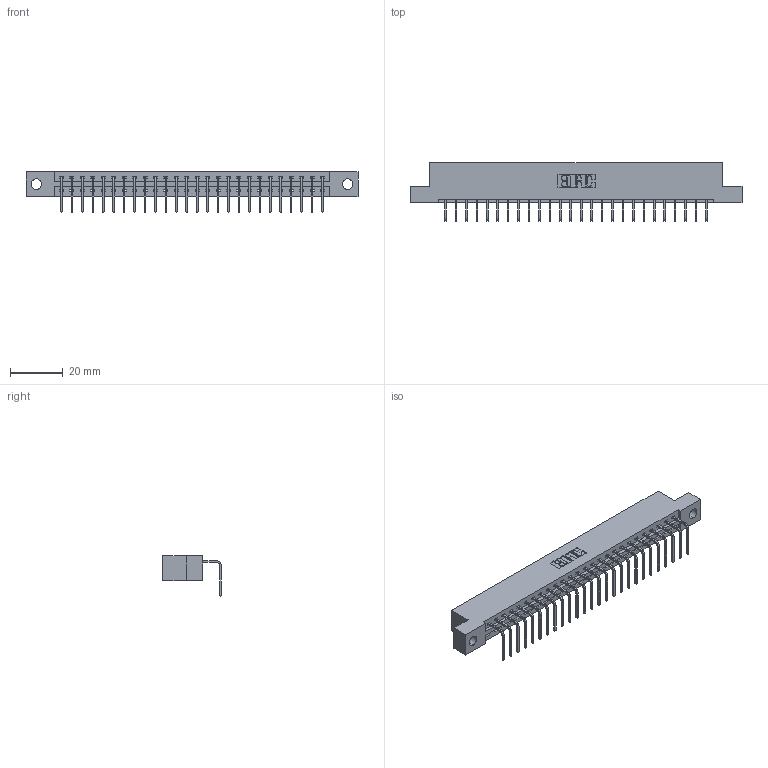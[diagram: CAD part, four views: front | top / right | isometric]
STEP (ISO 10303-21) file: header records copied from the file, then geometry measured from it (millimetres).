
FILE_DESCRIPTION (( 'STEP AP203' ), '1' );
FILE_NAME ('387-026-558-104.STEP', '2019-10-07T18:46:04', ( '' ), ( '' ), 'SwSTEP 2.0', 'SolidWorks 2016', '' );
FILE_SCHEMA (( 'CONFIG_CONTROL_DESIGN' ));
Length unit declared in the file: inch
Products named in the file (3): 337 Part_Flush Mounting Lugs - 0.156 Dia-TH; 345-292-001_558 Tail - 2; 387-026-558-104
Assembly tree (27 placements, depth 2):
  387-026-558-104
    337 Part_Flush Mounting Lugs - 0.156 Dia-TH
    345-292-001_558 Tail - 2  x26
Bounding box: 126.03 x 22.17 x 15.37 mm (x, y, z)
Volume: 12897.8 mm3; surface area: 13566.6 mm2
Topology: 27 solids, 27 shells, 1778 faces, 5355 edges, 3534 vertices
Faces by surface type: plane 1318, cylinder 460
Entity records: 21483 total; most frequent: CARTESIAN_POINT 3748, ORIENTED_EDGE 3710, DIRECTION 3187, EDGE_CURVE 1855, LINE 1727, VECTOR 1727, VERTEX_POINT 1234, AXIS2_PLACEMENT_3D 730
